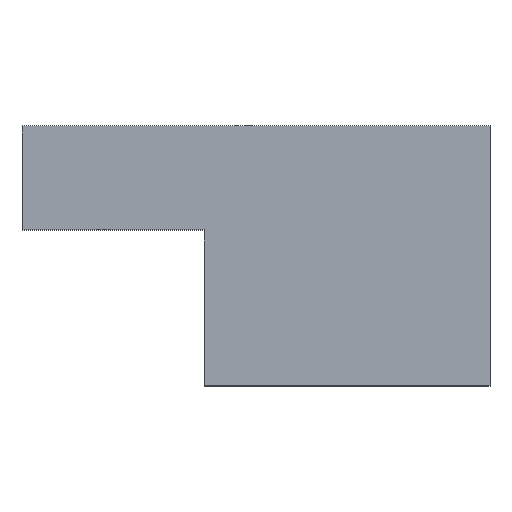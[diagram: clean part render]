
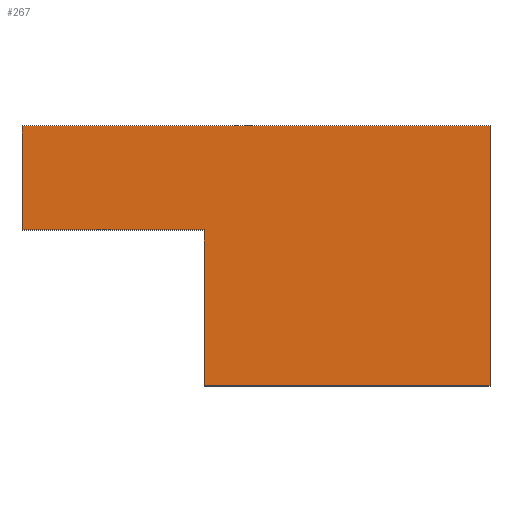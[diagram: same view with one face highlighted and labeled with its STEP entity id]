
A CAD part, top view. The second image highlights one B-rep face of the part: STEP entity #267.
In plain terms, the highlighted planar face has unit normal (0, 0, 1).
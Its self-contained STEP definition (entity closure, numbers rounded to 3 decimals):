
#83=CARTESIAN_POINT('',(0.0,0.0,3.0));
#84=VERTEX_POINT('',#83);
#91=CARTESIAN_POINT('',(18.,0.,3.0));
#92=VERTEX_POINT('',#91);
#93=CARTESIAN_POINT('',(18.,0.,3.0));
#94=DIRECTION('',(-1.0,0.0,0.0));
#95=VECTOR('',#94,18.);
#96=LINE('',#93,#95);
#97=EDGE_CURVE('',#92,#84,#96,.T.);
#122=CARTESIAN_POINT('',(18.,-10.,3.0));
#123=VERTEX_POINT('',#122);
#124=CARTESIAN_POINT('',(18.,-10.,3.0));
#125=DIRECTION('',(0.0,1.0,0.0));
#126=VECTOR('',#125,10.0);
#127=LINE('',#124,#126);
#128=EDGE_CURVE('',#123,#92,#127,.T.);
#153=CARTESIAN_POINT('',(7.,-10.,3.0));
#154=VERTEX_POINT('',#153);
#155=CARTESIAN_POINT('',(7.,-10.,3.0));
#156=DIRECTION('',(1.0,0.0,0.0));
#157=VECTOR('',#156,11.0);
#158=LINE('',#155,#157);
#159=EDGE_CURVE('',#154,#123,#158,.T.);
#184=CARTESIAN_POINT('',(7.,-4.,3.0));
#185=VERTEX_POINT('',#184);
#186=CARTESIAN_POINT('',(7.,-4.,3.0));
#187=DIRECTION('',(0.0,-1.0,0.0));
#188=VECTOR('',#187,6.);
#189=LINE('',#186,#188);
#190=EDGE_CURVE('',#185,#154,#189,.T.);
#215=CARTESIAN_POINT('',(0.0,-4.0,3.0));
#216=VERTEX_POINT('',#215);
#217=CARTESIAN_POINT('',(0.0,-4.0,3.0));
#218=DIRECTION('',(1.0,0.0,0.0));
#219=VECTOR('',#218,7.);
#220=LINE('',#217,#219);
#221=EDGE_CURVE('',#216,#185,#220,.T.);
#244=CARTESIAN_POINT('',(0.0,0.0,3.0));
#245=DIRECTION('',(0.0,-1.0,0.0));
#246=VECTOR('',#245,4.0);
#247=LINE('',#244,#246);
#248=EDGE_CURVE('',#84,#216,#247,.T.);
#254=CARTESIAN_POINT('',(9.75,-4.25,3.0));
#255=DIRECTION('',(0.0,0.0,1.0));
#256=DIRECTION('',(1.0,0.0,0.0));
#257=AXIS2_PLACEMENT_3D('',#254,#255,#256);
#258=PLANE('',#257);
#259=ORIENTED_EDGE('',*,*,#248,.T.);
#260=ORIENTED_EDGE('',*,*,#221,.T.);
#261=ORIENTED_EDGE('',*,*,#190,.T.);
#262=ORIENTED_EDGE('',*,*,#159,.T.);
#263=ORIENTED_EDGE('',*,*,#128,.T.);
#264=ORIENTED_EDGE('',*,*,#97,.T.);
#265=EDGE_LOOP('',(#259,#260,#261,#262,#263,#264));
#266=FACE_OUTER_BOUND('',#265,.T.);
#267=ADVANCED_FACE('',(#266),#258,.T.);
